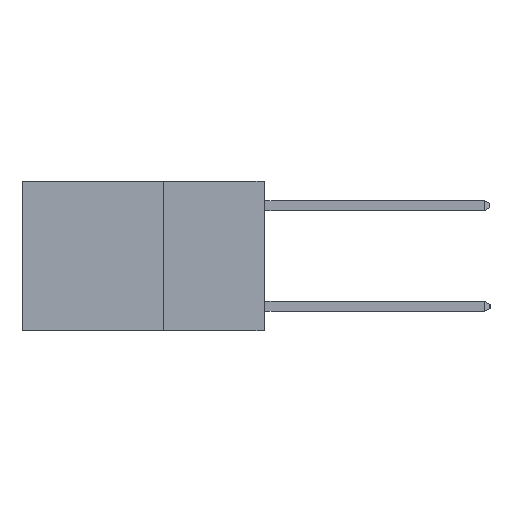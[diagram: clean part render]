
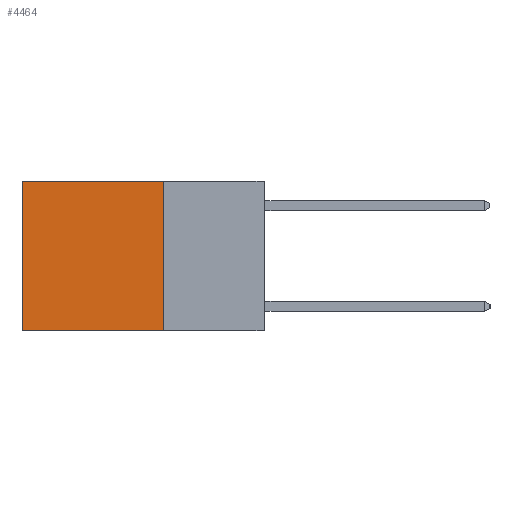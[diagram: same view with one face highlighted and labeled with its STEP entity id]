
A CAD part, left-side view. The second image highlights one B-rep face of the part: STEP entity #4464.
In plain terms, the highlighted planar face has unit normal (-1, 0, 0).
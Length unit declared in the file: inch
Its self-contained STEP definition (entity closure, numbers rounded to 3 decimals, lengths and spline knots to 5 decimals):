
#148 = LINE ( 'NONE', #10037, #11629 ) ;
#452 = CARTESIAN_POINT ( 'NONE',  ( 0.2625, 0.6, 0. ) ) ;
#790 = CARTESIAN_POINT ( 'NONE',  ( 0.2625, 0.25, 0. ) ) ;
#799 = EDGE_CURVE ( 'NONE', #4397, #8254, #148, .T. ) ;
#809 = FACE_OUTER_BOUND ( 'NONE', #7769, .T. ) ;
#952 = ORIENTED_EDGE ( 'NONE', *, *, #9690, .T. ) ;
#1693 = LINE ( 'NONE', #790, #8432 ) ;
#1700 = DIRECTION ( 'NONE',  ( 0., 1., 0. ) ) ;
#1932 = VECTOR ( 'NONE', #4122, 39.37008 ) ;
#2347 = DIRECTION ( 'NONE',  ( 0., 1., 0. ) ) ;
#3063 = EDGE_CURVE ( 'NONE', #3148, #10624, #4345, .T. ) ;
#3148 = VERTEX_POINT ( 'NONE', #7969 ) ;
#3431 = EDGE_CURVE ( 'NONE', #10624, #8254, #11284, .T. ) ;
#3745 = VECTOR ( 'NONE', #2347, 39.37008 ) ;
#4122 = DIRECTION ( 'NONE',  ( 0., 0., -1. ) ) ;
#4206 = CARTESIAN_POINT ( 'NONE',  ( 0.2625, 0.25, 0. ) ) ;
#4345 = LINE ( 'NONE', #7820, #1932 ) ;
#4397 = VERTEX_POINT ( 'NONE', #452 ) ;
#4464 = ADVANCED_FACE ( 'NONE', ( #809 ), #8798, .F. ) ;
#5176 = DIRECTION ( 'NONE',  ( 0., 0., -1. ) ) ;
#6932 = CARTESIAN_POINT ( 'NONE',  ( 0.2625, 0.25, -0.37 ) ) ;
#6933 = ORIENTED_EDGE ( 'NONE', *, *, #3431, .F. ) ;
#7266 = CARTESIAN_POINT ( 'NONE',  ( 0.2625, 0.25, -0.37 ) ) ;
#7685 = AXIS2_PLACEMENT_3D ( 'NONE', #4206, #10597, #5176 ) ;
#7769 = EDGE_LOOP ( 'NONE', ( #10421, #6933, #8534, #952 ) ) ;
#7820 = CARTESIAN_POINT ( 'NONE',  ( 0.2625, 0.25, 0. ) ) ;
#7969 = CARTESIAN_POINT ( 'NONE',  ( 0.2625, 0.25, 0. ) ) ;
#8254 = VERTEX_POINT ( 'NONE', #10090 ) ;
#8432 = VECTOR ( 'NONE', #1700, 39.37008 ) ;
#8534 = ORIENTED_EDGE ( 'NONE', *, *, #3063, .F. ) ;
#8798 = PLANE ( 'NONE',  #7685 ) ;
#9690 = EDGE_CURVE ( 'NONE', #3148, #4397, #1693, .T. ) ;
#10037 = CARTESIAN_POINT ( 'NONE',  ( 0.2625, 0.6, 0. ) ) ;
#10090 = CARTESIAN_POINT ( 'NONE',  ( 0.2625, 0.6, -0.37 ) ) ;
#10421 = ORIENTED_EDGE ( 'NONE', *, *, #799, .T. ) ;
#10597 = DIRECTION ( 'NONE',  ( 1., 0., 0. ) ) ;
#10624 = VERTEX_POINT ( 'NONE', #7266 ) ;
#10940 = DIRECTION ( 'NONE',  ( 0., 0., -1. ) ) ;
#11284 = LINE ( 'NONE', #6932, #3745 ) ;
#11629 = VECTOR ( 'NONE', #10940, 39.37008 ) ;
